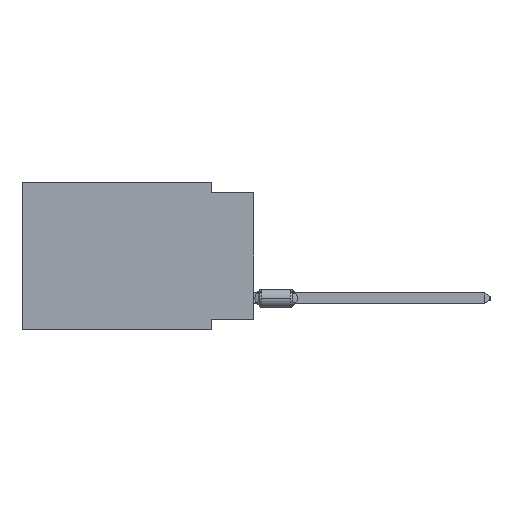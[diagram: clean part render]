
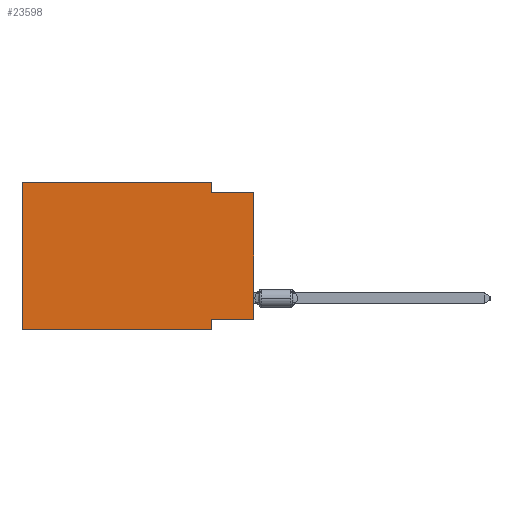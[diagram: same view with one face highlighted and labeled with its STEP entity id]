
A CAD part, left-side view. The second image highlights one B-rep face of the part: STEP entity #23598.
In plain terms, the highlighted planar face has unit normal (-1, 0, 0).
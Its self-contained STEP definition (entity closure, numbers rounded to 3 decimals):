
#378 = AXIS2_PLACEMENT_3D ( 'NONE', #4289, #26601, #9443 ) ;
#405 = VERTEX_POINT ( 'NONE', #14719 ) ;
#718 = EDGE_CURVE ( 'NONE', #10579, #21560, #8749, .T. ) ;
#2011 = DIRECTION ( 'NONE',  ( 0., -1., 0. ) ) ;
#2477 = CARTESIAN_POINT ( 'NONE',  ( 0., 2.54, -8.89 ) ) ;
#3480 = ORIENTED_EDGE ( 'NONE', *, *, #30814, .T. ) ;
#4113 = CARTESIAN_POINT ( 'NONE',  ( 0., 13.97, 0. ) ) ;
#4289 = CARTESIAN_POINT ( 'NONE',  ( 0., 13.97, 0. ) ) ;
#4358 = LINE ( 'NONE', #23769, #18139 ) ;
#5447 = EDGE_LOOP ( 'NONE', ( #3480, #7248, #14257, #12868, #15212, #10239, #30351, #9093 ) ) ;
#5657 = CARTESIAN_POINT ( 'NONE',  ( 0., 0., -8.255 ) ) ;
#5858 = CARTESIAN_POINT ( 'NONE',  ( 0., 2.54, 0. ) ) ;
#6713 = DIRECTION ( 'NONE',  ( 0., -1., 0. ) ) ;
#6984 = CARTESIAN_POINT ( 'NONE',  ( 0., 2.54, -0.635 ) ) ;
#7248 = ORIENTED_EDGE ( 'NONE', *, *, #23661, .F. ) ;
#7968 = VERTEX_POINT ( 'NONE', #16059 ) ;
#8008 = LINE ( 'NONE', #17877, #26154 ) ;
#8749 = LINE ( 'NONE', #20884, #22333 ) ;
#9093 = ORIENTED_EDGE ( 'NONE', *, *, #14561, .F. ) ;
#9134 = CARTESIAN_POINT ( 'NONE',  ( 0., 0., -0.635 ) ) ;
#9443 = DIRECTION ( 'NONE',  ( 0., 0., -1. ) ) ;
#9478 = VECTOR ( 'NONE', #16665, 1000. ) ;
#9622 = EDGE_CURVE ( 'NONE', #7968, #22917, #17636, .T. ) ;
#10239 = ORIENTED_EDGE ( 'NONE', *, *, #24846, .T. ) ;
#10579 = VERTEX_POINT ( 'NONE', #12040 ) ;
#10892 = CARTESIAN_POINT ( 'NONE',  ( 0., 2.54, 0. ) ) ;
#11201 = LINE ( 'NONE', #10892, #20172 ) ;
#11717 = FACE_OUTER_BOUND ( 'NONE', #5447, .T. ) ;
#12009 = CARTESIAN_POINT ( 'NONE',  ( 0., 2.54, -8.89 ) ) ;
#12040 = CARTESIAN_POINT ( 'NONE',  ( 0., 13.97, -8.89 ) ) ;
#12868 = ORIENTED_EDGE ( 'NONE', *, *, #19483, .F. ) ;
#13415 = VECTOR ( 'NONE', #29804, 1000. ) ;
#14128 = EDGE_CURVE ( 'NONE', #16535, #23999, #11201, .T. ) ;
#14257 = ORIENTED_EDGE ( 'NONE', *, *, #14128, .F. ) ;
#14561 = EDGE_CURVE ( 'NONE', #27885, #7968, #4358, .T. ) ;
#14719 = CARTESIAN_POINT ( 'NONE',  ( 0., 0., -0.635 ) ) ;
#15212 = ORIENTED_EDGE ( 'NONE', *, *, #718, .F. ) ;
#16059 = CARTESIAN_POINT ( 'NONE',  ( 0., 2.54, -8.255 ) ) ;
#16535 = VERTEX_POINT ( 'NONE', #5858 ) ;
#16665 = DIRECTION ( 'NONE',  ( 0., 0., 1. ) ) ;
#16722 = CARTESIAN_POINT ( 'NONE',  ( 0., 13.97, -8.89 ) ) ;
#17636 = LINE ( 'NONE', #2477, #13415 ) ;
#17877 = CARTESIAN_POINT ( 'NONE',  ( 0., 13.97, 0. ) ) ;
#18139 = VECTOR ( 'NONE', #31518, 1000. ) ;
#18628 = DIRECTION ( 'NONE',  ( 0., 0., -1. ) ) ;
#18992 = PLANE ( 'NONE',  #378 ) ;
#19483 = EDGE_CURVE ( 'NONE', #21560, #16535, #8008, .T. ) ;
#20172 = VECTOR ( 'NONE', #18628, 1000. ) ;
#20884 = CARTESIAN_POINT ( 'NONE',  ( 0., 13.97, 0. ) ) ;
#21218 = LINE ( 'NONE', #31406, #9478 ) ;
#21560 = VERTEX_POINT ( 'NONE', #4113 ) ;
#22075 = VECTOR ( 'NONE', #6713, 1000. ) ;
#22333 = VECTOR ( 'NONE', #26228, 1000. ) ;
#22885 = DIRECTION ( 'NONE',  ( 0., -1., 0. ) ) ;
#22917 = VERTEX_POINT ( 'NONE', #12009 ) ;
#23598 = ADVANCED_FACE ( 'NONE', ( #11717 ), #18992, .F. ) ;
#23661 = EDGE_CURVE ( 'NONE', #23999, #405, #31290, .T. ) ;
#23769 = CARTESIAN_POINT ( 'NONE',  ( 0., 0., -8.255 ) ) ;
#23999 = VERTEX_POINT ( 'NONE', #6984 ) ;
#24846 = EDGE_CURVE ( 'NONE', #10579, #22917, #28726, .T. ) ;
#26154 = VECTOR ( 'NONE', #22885, 1000. ) ;
#26228 = DIRECTION ( 'NONE',  ( 0., 0., 1. ) ) ;
#26601 = DIRECTION ( 'NONE',  ( 1., 0., 0. ) ) ;
#27885 = VERTEX_POINT ( 'NONE', #5657 ) ;
#28726 = LINE ( 'NONE', #16722, #22075 ) ;
#29804 = DIRECTION ( 'NONE',  ( 0., 0., -1. ) ) ;
#30351 = ORIENTED_EDGE ( 'NONE', *, *, #9622, .F. ) ;
#30814 = EDGE_CURVE ( 'NONE', #27885, #405, #21218, .T. ) ;
#31290 = LINE ( 'NONE', #9134, #31879 ) ;
#31406 = CARTESIAN_POINT ( 'NONE',  ( 0., 0., 0. ) ) ;
#31518 = DIRECTION ( 'NONE',  ( 0., 1., 0. ) ) ;
#31879 = VECTOR ( 'NONE', #2011, 1000. ) ;
